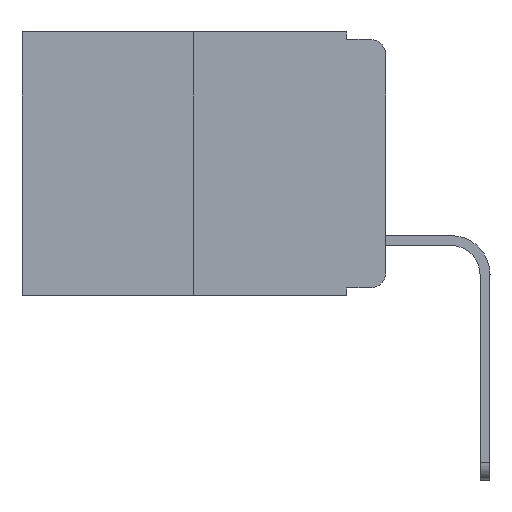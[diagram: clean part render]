
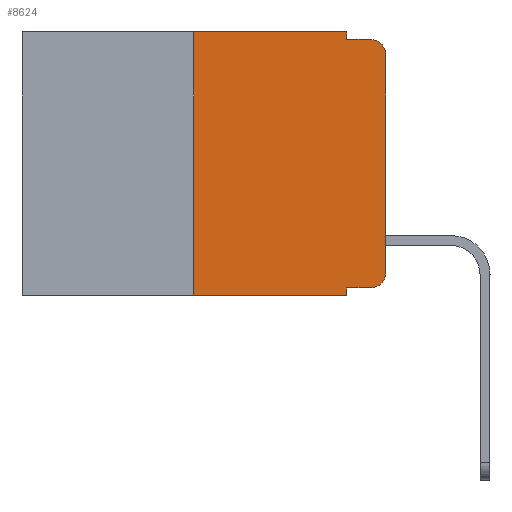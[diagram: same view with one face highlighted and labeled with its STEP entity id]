
A CAD part, left-side view. The second image highlights one B-rep face of the part: STEP entity #8624.
In plain terms, the highlighted planar face has unit normal (-1, 0, 0).
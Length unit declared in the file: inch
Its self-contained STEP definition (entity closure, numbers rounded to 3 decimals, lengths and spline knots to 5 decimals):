
#15 = LINE ( 'NONE', #5797, #7740 ) ;
#91 = VERTEX_POINT ( 'NONE', #3521 ) ;
#135 = CARTESIAN_POINT ( 'NONE',  ( 0., 0.473, 0. ) ) ;
#226 = DIRECTION ( 'NONE',  ( 0., 0., 1. ) ) ;
#402 = CARTESIAN_POINT ( 'NONE',  ( 0., 0., -0.03 ) ) ;
#419 = ORIENTED_EDGE ( 'NONE', *, *, #2377, .T. ) ;
#446 = DIRECTION ( 'NONE',  ( -1., 0., 0. ) ) ;
#512 = PLANE ( 'NONE',  #1049 ) ;
#545 = EDGE_CURVE ( 'NONE', #2145, #1074, #2046, .T. ) ;
#669 = CARTESIAN_POINT ( 'NONE',  ( 0., 0.051, -0.333 ) ) ;
#893 = CARTESIAN_POINT ( 'NONE',  ( 0., 0.051, 0. ) ) ;
#1049 = AXIS2_PLACEMENT_3D ( 'NONE', #1274, #8798, #2840 ) ;
#1074 = VERTEX_POINT ( 'NONE', #8652 ) ;
#1090 = VECTOR ( 'NONE', #7292, 39.37008 ) ;
#1274 = CARTESIAN_POINT ( 'NONE',  ( 0., 0.473, 0. ) ) ;
#1422 = VECTOR ( 'NONE', #8684, 39.37008 ) ;
#1503 = ORIENTED_EDGE ( 'NONE', *, *, #8281, .F. ) ;
#1585 = VERTEX_POINT ( 'NONE', #6417 ) ;
#1827 = EDGE_CURVE ( 'NONE', #7812, #2145, #5316, .T. ) ;
#2046 = CIRCLE ( 'NONE', #4631, 0.02 ) ;
#2145 = VERTEX_POINT ( 'NONE', #8580 ) ;
#2374 = CARTESIAN_POINT ( 'NONE',  ( 0., 0., 0. ) ) ;
#2377 = EDGE_CURVE ( 'NONE', #91, #1585, #15, .T. ) ;
#2500 = ORIENTED_EDGE ( 'NONE', *, *, #6449, .F. ) ;
#2684 = VECTOR ( 'NONE', #4573, 39.37008 ) ;
#2840 = DIRECTION ( 'NONE',  ( 0., 0., -1. ) ) ;
#3081 = VERTEX_POINT ( 'NONE', #7603 ) ;
#3276 = CARTESIAN_POINT ( 'NONE',  ( 0., 0.051, -0.333 ) ) ;
#3293 = CARTESIAN_POINT ( 'NONE',  ( 0., 0.051, -0.01 ) ) ;
#3379 = ORIENTED_EDGE ( 'NONE', *, *, #5436, .F. ) ;
#3407 = DIRECTION ( 'NONE',  ( 0., 0., -1. ) ) ;
#3521 = CARTESIAN_POINT ( 'NONE',  ( 0., 0.25, -0.343 ) ) ;
#4190 = LINE ( 'NONE', #6041, #4789 ) ;
#4245 = DIRECTION ( 'NONE',  ( 0., -1., 0. ) ) ;
#4249 = CARTESIAN_POINT ( 'NONE',  ( 0., 0.051, 0. ) ) ;
#4573 = DIRECTION ( 'NONE',  ( 0., 0., -1. ) ) ;
#4607 = CARTESIAN_POINT ( 'NONE',  ( 0., 0.051, 0. ) ) ;
#4631 = AXIS2_PLACEMENT_3D ( 'NONE', #7163, #6444, #3407 ) ;
#4772 = LINE ( 'NONE', #6549, #6501 ) ;
#4789 = VECTOR ( 'NONE', #6180, 39.37008 ) ;
#5187 = VECTOR ( 'NONE', #226, 39.37008 ) ;
#5311 = LINE ( 'NONE', #4607, #2684 ) ;
#5316 = LINE ( 'NONE', #669, #1090 ) ;
#5436 = EDGE_CURVE ( 'NONE', #91, #6954, #4190, .T. ) ;
#5462 = DIRECTION ( 'NONE',  ( 0., -1., 0. ) ) ;
#5684 = LINE ( 'NONE', #135, #8462 ) ;
#5691 = EDGE_LOOP ( 'NONE', ( #7018, #9182, #2500, #1503, #7201, #3379, #419, #7189, #9490, #6270 ) ) ;
#5797 = CARTESIAN_POINT ( 'NONE',  ( 0., 0.473, -0.343 ) ) ;
#5907 = CIRCLE ( 'NONE', #6480, 0.02 ) ;
#6041 = CARTESIAN_POINT ( 'NONE',  ( 0., 0.25, 0. ) ) ;
#6180 = DIRECTION ( 'NONE',  ( 0., 0., 1. ) ) ;
#6270 = ORIENTED_EDGE ( 'NONE', *, *, #545, .T. ) ;
#6337 = VERTEX_POINT ( 'NONE', #402 ) ;
#6417 = CARTESIAN_POINT ( 'NONE',  ( 0., 0.051, -0.343 ) ) ;
#6424 = DIRECTION ( 'NONE',  ( 0., 0., -1. ) ) ;
#6444 = DIRECTION ( 'NONE',  ( -1., 0., 0. ) ) ;
#6449 = EDGE_CURVE ( 'NONE', #8393, #3081, #4772, .T. ) ;
#6480 = AXIS2_PLACEMENT_3D ( 'NONE', #8634, #446, #6424 ) ;
#6501 = VECTOR ( 'NONE', #4245, 39.37008 ) ;
#6549 = CARTESIAN_POINT ( 'NONE',  ( 0., 0.051, -0.01 ) ) ;
#6954 = VERTEX_POINT ( 'NONE', #9520 ) ;
#6958 = EDGE_CURVE ( 'NONE', #6337, #3081, #5907, .T. ) ;
#7018 = ORIENTED_EDGE ( 'NONE', *, *, #9594, .T. ) ;
#7153 = LINE ( 'NONE', #2374, #5187 ) ;
#7163 = CARTESIAN_POINT ( 'NONE',  ( 0., 0.02, -0.313 ) ) ;
#7189 = ORIENTED_EDGE ( 'NONE', *, *, #9153, .F. ) ;
#7201 = ORIENTED_EDGE ( 'NONE', *, *, #7267, .F. ) ;
#7267 = EDGE_CURVE ( 'NONE', #6954, #9509, #5684, .T. ) ;
#7292 = DIRECTION ( 'NONE',  ( 0., -1., 0. ) ) ;
#7345 = DIRECTION ( 'NONE',  ( 0., -1., 0. ) ) ;
#7603 = CARTESIAN_POINT ( 'NONE',  ( 0., 0.02, -0.01 ) ) ;
#7612 = LINE ( 'NONE', #4249, #1422 ) ;
#7740 = VECTOR ( 'NONE', #7345, 39.37008 ) ;
#7812 = VERTEX_POINT ( 'NONE', #3276 ) ;
#8281 = EDGE_CURVE ( 'NONE', #9509, #8393, #5311, .T. ) ;
#8393 = VERTEX_POINT ( 'NONE', #3293 ) ;
#8462 = VECTOR ( 'NONE', #5462, 39.37008 ) ;
#8580 = CARTESIAN_POINT ( 'NONE',  ( 0., 0.02, -0.333 ) ) ;
#8624 = ADVANCED_FACE ( 'NONE', ( #8780 ), #512, .F. ) ;
#8634 = CARTESIAN_POINT ( 'NONE',  ( 0., 0.02, -0.03 ) ) ;
#8652 = CARTESIAN_POINT ( 'NONE',  ( 0., 0., -0.313 ) ) ;
#8684 = DIRECTION ( 'NONE',  ( 0., 0., -1. ) ) ;
#8780 = FACE_OUTER_BOUND ( 'NONE', #5691, .T. ) ;
#8798 = DIRECTION ( 'NONE',  ( 1., 0., 0. ) ) ;
#9153 = EDGE_CURVE ( 'NONE', #7812, #1585, #7612, .T. ) ;
#9182 = ORIENTED_EDGE ( 'NONE', *, *, #6958, .T. ) ;
#9490 = ORIENTED_EDGE ( 'NONE', *, *, #1827, .T. ) ;
#9509 = VERTEX_POINT ( 'NONE', #893 ) ;
#9520 = CARTESIAN_POINT ( 'NONE',  ( 0., 0.25, 0. ) ) ;
#9594 = EDGE_CURVE ( 'NONE', #1074, #6337, #7153, .T. ) ;
